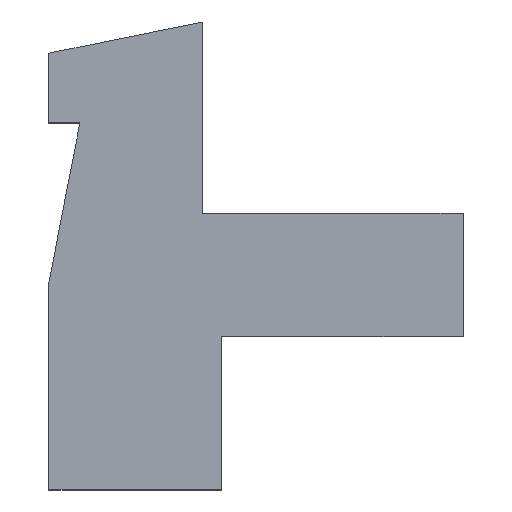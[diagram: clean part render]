
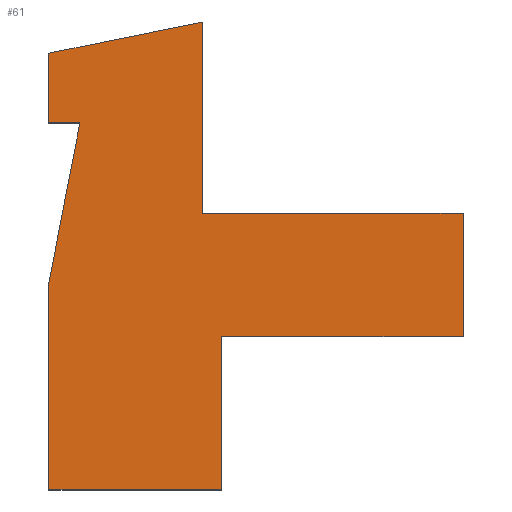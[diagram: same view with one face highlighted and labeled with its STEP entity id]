
A CAD part, top view. The second image highlights one B-rep face of the part: STEP entity #61.
In plain terms, the highlighted planar face has unit normal (0, 0, 1).
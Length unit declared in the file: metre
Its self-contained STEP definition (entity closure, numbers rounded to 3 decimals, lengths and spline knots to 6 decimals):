
#61=ADVANCED_FACE('0:71305',(#94),#95,.T.);
#94=FACE_OUTER_BOUND('',#135,.T.);
#95=PLANE('',#136);
#135=EDGE_LOOP('',(#237,#238,#239,#240,#241,#242,#243,#244,#245,#246,#247,#248,#249));
#136=AXIS2_PLACEMENT_3D('',#250,#251,#252);
#237=ORIENTED_EDGE('',*,*,#325,.F.);
#238=ORIENTED_EDGE('',*,*,#330,.T.);
#239=ORIENTED_EDGE('',*,*,#333,.T.);
#240=ORIENTED_EDGE('',*,*,#345,.T.);
#241=ORIENTED_EDGE('',*,*,#322,.T.);
#242=ORIENTED_EDGE('',*,*,#346,.T.);
#243=ORIENTED_EDGE('',*,*,#347,.F.);
#244=ORIENTED_EDGE('',*,*,#348,.F.);
#245=ORIENTED_EDGE('',*,*,#349,.T.);
#246=ORIENTED_EDGE('',*,*,#350,.T.);
#247=ORIENTED_EDGE('',*,*,#351,.T.);
#248=ORIENTED_EDGE('',*,*,#352,.T.);
#249=ORIENTED_EDGE('',*,*,#343,.F.);
#250=CARTESIAN_POINT('',(-0.011837,-0.008414,0.006));
#251=DIRECTION('',(0.0,0.0,1.0));
#252=DIRECTION('',(1.0,0.0,0.0));
#322=EDGE_CURVE('0:71350',#380,#378,#381,.F.);
#325=EDGE_CURVE('0:71359',#383,#386,#387,.F.);
#330=EDGE_CURVE('0:71374',#383,#393,#395,.T.);
#333=EDGE_CURVE('0:71383',#393,#398,#400,.F.);
#343=EDGE_CURVE('0:71413',#386,#417,#418,.T.);
#345=EDGE_CURVE('0:71419',#398,#380,#420,.T.);
#346=EDGE_CURVE('0:71422',#378,#421,#422,.T.);
#347=EDGE_CURVE('0:71425',#423,#421,#424,.T.);
#348=EDGE_CURVE('0:71428',#425,#423,#426,.T.);
#349=EDGE_CURVE('0:71431',#425,#427,#428,.T.);
#350=EDGE_CURVE('0:71434',#427,#429,#430,.T.);
#351=EDGE_CURVE('0:71437',#429,#431,#432,.T.);
#352=EDGE_CURVE('0:71440',#431,#417,#433,.T.);
#378=VERTEX_POINT('',#464);
#380=VERTEX_POINT('',#467);
#381=LINE('',#468,#469);
#383=VERTEX_POINT('',#472);
#386=VERTEX_POINT('',#476);
#387=LINE('',#477,#478);
#393=VERTEX_POINT('',#487);
#395=LINE('',#490,#491);
#398=VERTEX_POINT('',#495);
#400=LINE('',#498,#499);
#417=VERTEX_POINT('',#525);
#418=LINE('',#526,#527);
#420=LINE('',#530,#531);
#421=VERTEX_POINT('',#532);
#422=LINE('',#533,#534);
#423=VERTEX_POINT('',#535);
#424=LINE('',#536,#537);
#425=VERTEX_POINT('',#538);
#426=LINE('',#539,#540);
#427=VERTEX_POINT('',#541);
#428=LINE('',#542,#543);
#429=VERTEX_POINT('',#544);
#430=LINE('',#545,#546);
#431=VERTEX_POINT('',#547);
#432=LINE('',#548,#549);
#433=LINE('',#550,#551);
#464=CARTESIAN_POINT('',(-0.020337,0.005586,0.006));
#467=CARTESIAN_POINT('',(-0.011837,0.005586,0.006));
#468=CARTESIAN_POINT('',(-0.016087,0.005586,0.006));
#469=VECTOR('',#588,0.0085);
#472=CARTESIAN_POINT('',(-0.0197,-0.003414,0.006));
#476=CARTESIAN_POINT('',(-0.025337,-0.003414,0.006));
#477=CARTESIAN_POINT('',(-0.018587,-0.003414,0.006));
#478=VECTOR('',#591,0.005637);
#487=CARTESIAN_POINT('',(-0.0197,0.001586,0.006));
#490=CARTESIAN_POINT('',(-0.0197,-0.020352,0.006));
#491=VECTOR('',#596,0.005);
#495=CARTESIAN_POINT('',(-0.011837,0.001586,0.006));
#498=CARTESIAN_POINT('',(-0.019581,0.001586,0.006));
#499=VECTOR('',#599,0.007863);
#525=CARTESIAN_POINT('',(-0.025337,0.003339,0.006));
#526=CARTESIAN_POINT('',(-0.025337,-0.008414,0.006));
#527=VECTOR('',#609,0.006753);
#530=CARTESIAN_POINT('',(-0.011837,-0.008414,0.006));
#531=VECTOR('',#611,0.004);
#532=CARTESIAN_POINT('',(-0.020337,0.011825,0.006));
#533=CARTESIAN_POINT('',(-0.020337,0.001836,0.006));
#534=VECTOR('',#612,0.006239);
#535=CARTESIAN_POINT('',(-0.025337,0.010807,0.006));
#536=CARTESIAN_POINT('',(-0.017476,0.012407,0.006));
#537=VECTOR('',#613,0.005102);
#538=CARTESIAN_POINT('',(-0.025337,0.008542,0.006));
#539=CARTESIAN_POINT('',(-0.025337,-0.008414,0.006));
#540=VECTOR('',#614,0.002265);
#541=CARTESIAN_POINT('',(-0.024326,0.008542,0.006));
#542=CARTESIAN_POINT('',(-0.025337,0.008542,0.006));
#543=VECTOR('',#615,0.001011);
#544=CARTESIAN_POINT('',(-0.024499,0.007643,0.006));
#545=CARTESIAN_POINT('',(-0.024326,0.008542,0.006));
#546=VECTOR('',#616,0.000916);
#547=CARTESIAN_POINT('',(-0.024719,0.006523,0.006));
#548=CARTESIAN_POINT('',(-0.024498,0.007643,0.006));
#549=VECTOR('',#617,0.001142);
#550=CARTESIAN_POINT('',(-0.024326,0.008542,0.006));
#551=VECTOR('',#618,0.003243);
#588=DIRECTION('',(1.0,0.0,0.0));
#591=DIRECTION('',(1.0,0.0,0.0));
#596=DIRECTION('',(0.,1.0,0.0));
#599=DIRECTION('',(-1.0,0.0,0.0));
#609=DIRECTION('',(0.0,1.0,0.0));
#611=DIRECTION('',(0.0,1.0,0.0));
#612=DIRECTION('',(0.0,1.0,0.0));
#613=DIRECTION('',(0.98,0.199,0.0));
#614=DIRECTION('',(0.0,1.0,0.0));
#615=DIRECTION('',(1.0,0.0,0.0));
#616=DIRECTION('',(-0.191,-0.982,0.));
#617=DIRECTION('',(-0.193,-0.981,0.));
#618=DIRECTION('',(-0.191,-0.982,0.));
